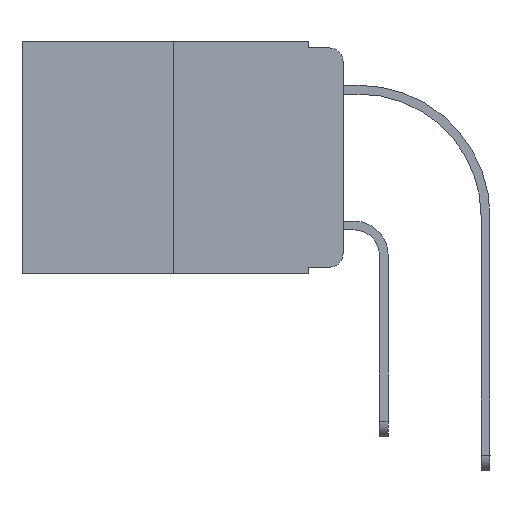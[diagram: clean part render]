
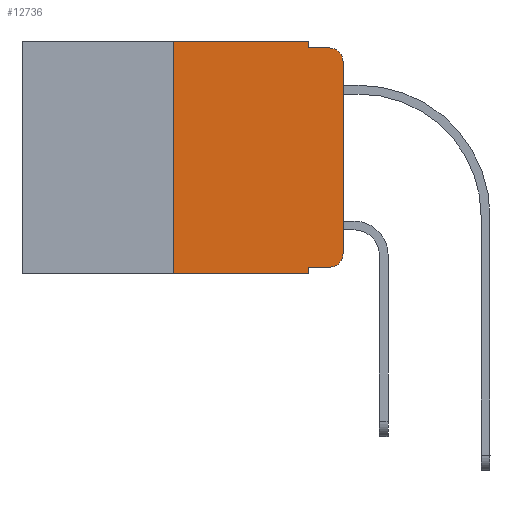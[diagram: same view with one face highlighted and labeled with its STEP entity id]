
A CAD part, left-side view. The second image highlights one B-rep face of the part: STEP entity #12736.
In plain terms, the highlighted planar face has unit normal (-1, 0, 0).
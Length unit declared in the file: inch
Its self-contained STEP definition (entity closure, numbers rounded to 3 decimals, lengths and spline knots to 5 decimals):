
#282 = LINE ( 'NONE', #13738, #4736 ) ;
#1094 = CARTESIAN_POINT ( 'NONE',  ( 0., 0.02, -0.313 ) ) ;
#1119 = DIRECTION ( 'NONE',  ( 0., 0., -1. ) ) ;
#1288 = CARTESIAN_POINT ( 'NONE',  ( 0., 0.051, 0. ) ) ;
#1579 = LINE ( 'NONE', #13552, #3128 ) ;
#1722 = VERTEX_POINT ( 'NONE', #6492 ) ;
#1785 = ORIENTED_EDGE ( 'NONE', *, *, #8238, .T. ) ;
#1835 = CARTESIAN_POINT ( 'NONE',  ( 0., 0.051, -0.01 ) ) ;
#2059 = ORIENTED_EDGE ( 'NONE', *, *, #14382, .T. ) ;
#2104 = DIRECTION ( 'NONE',  ( 0., -1., 0. ) ) ;
#2285 = CARTESIAN_POINT ( 'NONE',  ( 0., 0.473, -0.343 ) ) ;
#2296 = EDGE_CURVE ( 'NONE', #2424, #12540, #15182, .T. ) ;
#2333 = CARTESIAN_POINT ( 'NONE',  ( 0., 0.02, -0.01 ) ) ;
#2418 = DIRECTION ( 'NONE',  ( 1., 0., 0. ) ) ;
#2424 = VERTEX_POINT ( 'NONE', #2547 ) ;
#2514 = VERTEX_POINT ( 'NONE', #15754 ) ;
#2547 = CARTESIAN_POINT ( 'NONE',  ( 0., 0., -0.03 ) ) ;
#2905 = EDGE_LOOP ( 'NONE', ( #4125, #4213, #3171, #6321, #10826, #7469, #2059, #16851, #11951, #1785 ) ) ;
#3128 = VECTOR ( 'NONE', #9601, 39.37008 ) ;
#3171 = ORIENTED_EDGE ( 'NONE', *, *, #5865, .F. ) ;
#3248 = LINE ( 'NONE', #1835, #6342 ) ;
#3268 = DIRECTION ( 'NONE',  ( -1., 0., 0. ) ) ;
#3739 = PLANE ( 'NONE',  #9191 ) ;
#4029 = DIRECTION ( 'NONE',  ( 0., 0., -1. ) ) ;
#4032 = VERTEX_POINT ( 'NONE', #9187 ) ;
#4125 = ORIENTED_EDGE ( 'NONE', *, *, #11013, .T. ) ;
#4213 = ORIENTED_EDGE ( 'NONE', *, *, #2296, .T. ) ;
#4368 = EDGE_CURVE ( 'NONE', #4032, #12181, #5433, .T. ) ;
#4391 = DIRECTION ( 'NONE',  ( 0., -1., 0. ) ) ;
#4430 = VERTEX_POINT ( 'NONE', #11019 ) ;
#4545 = DIRECTION ( 'NONE',  ( 0., 0., 1. ) ) ;
#4736 = VECTOR ( 'NONE', #5817, 39.37008 ) ;
#5433 = LINE ( 'NONE', #1288, #12637 ) ;
#5817 = DIRECTION ( 'NONE',  ( 0., -1., 0. ) ) ;
#5865 = EDGE_CURVE ( 'NONE', #1722, #12540, #3248, .T. ) ;
#6089 = DIRECTION ( 'NONE',  ( 0., 0., -1. ) ) ;
#6321 = ORIENTED_EDGE ( 'NONE', *, *, #9712, .F. ) ;
#6342 = VECTOR ( 'NONE', #4391, 39.37008 ) ;
#6408 = CIRCLE ( 'NONE', #13698, 0.02 ) ;
#6485 = LINE ( 'NONE', #13179, #11392 ) ;
#6492 = CARTESIAN_POINT ( 'NONE',  ( 0., 0.051, -0.01 ) ) ;
#6701 = VECTOR ( 'NONE', #2104, 39.37008 ) ;
#6922 = EDGE_CURVE ( 'NONE', #8266, #10216, #1579, .T. ) ;
#7024 = CARTESIAN_POINT ( 'NONE',  ( 0., 0., 0. ) ) ;
#7469 = ORIENTED_EDGE ( 'NONE', *, *, #10117, .F. ) ;
#7794 = LINE ( 'NONE', #17009, #10561 ) ;
#7957 = CARTESIAN_POINT ( 'NONE',  ( 0., 0.25, 0. ) ) ;
#8049 = DIRECTION ( 'NONE',  ( 0., 0., -1. ) ) ;
#8238 = EDGE_CURVE ( 'NONE', #4430, #8707, #6408, .T. ) ;
#8266 = VERTEX_POINT ( 'NONE', #7957 ) ;
#8707 = VERTEX_POINT ( 'NONE', #14271 ) ;
#8965 = EDGE_CURVE ( 'NONE', #4032, #4430, #282, .T. ) ;
#9187 = CARTESIAN_POINT ( 'NONE',  ( 0., 0.051, -0.333 ) ) ;
#9191 = AXIS2_PLACEMENT_3D ( 'NONE', #14729, #2418, #8049 ) ;
#9601 = DIRECTION ( 'NONE',  ( 0., -1., 0. ) ) ;
#9712 = EDGE_CURVE ( 'NONE', #10216, #1722, #6485, .T. ) ;
#10051 = CARTESIAN_POINT ( 'NONE',  ( 0., 0.02, -0.03 ) ) ;
#10117 = EDGE_CURVE ( 'NONE', #2514, #8266, #7794, .T. ) ;
#10216 = VERTEX_POINT ( 'NONE', #16456 ) ;
#10413 = AXIS2_PLACEMENT_3D ( 'NONE', #10051, #3268, #6089 ) ;
#10439 = FACE_OUTER_BOUND ( 'NONE', #2905, .T. ) ;
#10561 = VECTOR ( 'NONE', #11831, 39.37008 ) ;
#10826 = ORIENTED_EDGE ( 'NONE', *, *, #6922, .F. ) ;
#10853 = DIRECTION ( 'NONE',  ( 0., 0., -1. ) ) ;
#11013 = EDGE_CURVE ( 'NONE', #8707, #2424, #16504, .T. ) ;
#11019 = CARTESIAN_POINT ( 'NONE',  ( 0., 0.02, -0.333 ) ) ;
#11392 = VECTOR ( 'NONE', #1119, 39.37008 ) ;
#11831 = DIRECTION ( 'NONE',  ( 0., 0., 1. ) ) ;
#11909 = DIRECTION ( 'NONE',  ( -1., 0., 0. ) ) ;
#11951 = ORIENTED_EDGE ( 'NONE', *, *, #8965, .T. ) ;
#12181 = VERTEX_POINT ( 'NONE', #15241 ) ;
#12540 = VERTEX_POINT ( 'NONE', #2333 ) ;
#12637 = VECTOR ( 'NONE', #4029, 39.37008 ) ;
#12736 = ADVANCED_FACE ( 'NONE', ( #10439 ), #3739, .F. ) ;
#13179 = CARTESIAN_POINT ( 'NONE',  ( 0., 0.051, 0. ) ) ;
#13552 = CARTESIAN_POINT ( 'NONE',  ( 0., 0.473, 0. ) ) ;
#13698 = AXIS2_PLACEMENT_3D ( 'NONE', #1094, #11909, #10853 ) ;
#13738 = CARTESIAN_POINT ( 'NONE',  ( 0., 0.051, -0.333 ) ) ;
#14159 = LINE ( 'NONE', #2285, #6701 ) ;
#14271 = CARTESIAN_POINT ( 'NONE',  ( 0., 0., -0.313 ) ) ;
#14382 = EDGE_CURVE ( 'NONE', #2514, #12181, #14159, .T. ) ;
#14729 = CARTESIAN_POINT ( 'NONE',  ( 0., 0.473, 0. ) ) ;
#15182 = CIRCLE ( 'NONE', #10413, 0.02 ) ;
#15241 = CARTESIAN_POINT ( 'NONE',  ( 0., 0.051, -0.343 ) ) ;
#15754 = CARTESIAN_POINT ( 'NONE',  ( 0., 0.25, -0.343 ) ) ;
#16139 = VECTOR ( 'NONE', #4545, 39.37008 ) ;
#16456 = CARTESIAN_POINT ( 'NONE',  ( 0., 0.051, 0. ) ) ;
#16504 = LINE ( 'NONE', #7024, #16139 ) ;
#16851 = ORIENTED_EDGE ( 'NONE', *, *, #4368, .F. ) ;
#17009 = CARTESIAN_POINT ( 'NONE',  ( 0., 0.25, 0. ) ) ;
